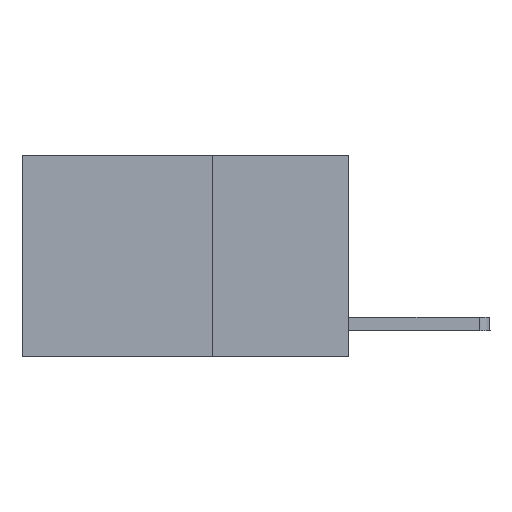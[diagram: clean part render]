
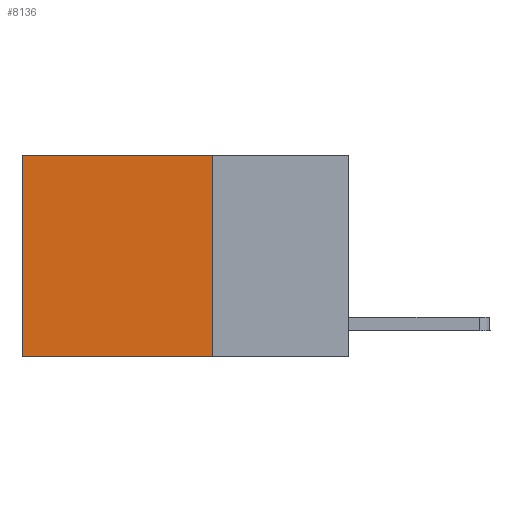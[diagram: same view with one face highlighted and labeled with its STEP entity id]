
A CAD part, left-side view. The second image highlights one B-rep face of the part: STEP entity #8136.
In plain terms, the highlighted planar face has unit normal (-1, 0, 0).
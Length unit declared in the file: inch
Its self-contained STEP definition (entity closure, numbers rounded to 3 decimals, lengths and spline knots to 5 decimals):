
#453 = ORIENTED_EDGE ( 'NONE', *, *, #1893, .F. ) ;
#514 = EDGE_CURVE ( 'NONE', #7480, #708, #1747, .T. ) ;
#708 = VERTEX_POINT ( 'NONE', #3586 ) ;
#758 = DIRECTION ( 'NONE',  ( 0., 1., 0. ) ) ;
#952 = CARTESIAN_POINT ( 'NONE',  ( 0.2625, 0.6, 0. ) ) ;
#1165 = VERTEX_POINT ( 'NONE', #2526 ) ;
#1647 = VERTEX_POINT ( 'NONE', #8555 ) ;
#1747 = LINE ( 'NONE', #3831, #3969 ) ;
#1850 = VECTOR ( 'NONE', #7423, 39.37008 ) ;
#1893 = EDGE_CURVE ( 'NONE', #1647, #1165, #5089, .T. ) ;
#1914 = CARTESIAN_POINT ( 'NONE',  ( 0.2625, 0.25, 0. ) ) ;
#2224 = LINE ( 'NONE', #7095, #2429 ) ;
#2429 = VECTOR ( 'NONE', #758, 39.37008 ) ;
#2526 = CARTESIAN_POINT ( 'NONE',  ( 0.2625, 0.25, -0.37 ) ) ;
#2721 = ORIENTED_EDGE ( 'NONE', *, *, #7191, .T. ) ;
#2847 = DIRECTION ( 'NONE',  ( 0., 0., -1. ) ) ;
#3586 = CARTESIAN_POINT ( 'NONE',  ( 0.2625, 0.6, -0.37 ) ) ;
#3684 = AXIS2_PLACEMENT_3D ( 'NONE', #4658, #7425, #4567 ) ;
#3831 = CARTESIAN_POINT ( 'NONE',  ( 0.2625, 0.6, 0. ) ) ;
#3880 = DIRECTION ( 'NONE',  ( 0., 0., -1. ) ) ;
#3969 = VECTOR ( 'NONE', #3880, 39.37008 ) ;
#4227 = ORIENTED_EDGE ( 'NONE', *, *, #8881, .F. ) ;
#4567 = DIRECTION ( 'NONE',  ( 0., 0., -1. ) ) ;
#4658 = CARTESIAN_POINT ( 'NONE',  ( 0.2625, 0.25, 0. ) ) ;
#5089 = LINE ( 'NONE', #5870, #6672 ) ;
#5213 = LINE ( 'NONE', #1914, #1850 ) ;
#5215 = FACE_OUTER_BOUND ( 'NONE', #6217, .T. ) ;
#5870 = CARTESIAN_POINT ( 'NONE',  ( 0.2625, 0.25, 0. ) ) ;
#6074 = ORIENTED_EDGE ( 'NONE', *, *, #514, .T. ) ;
#6217 = EDGE_LOOP ( 'NONE', ( #6074, #4227, #453, #2721 ) ) ;
#6672 = VECTOR ( 'NONE', #2847, 39.37008 ) ;
#7095 = CARTESIAN_POINT ( 'NONE',  ( 0.2625, 0.25, -0.37 ) ) ;
#7191 = EDGE_CURVE ( 'NONE', #1647, #7480, #5213, .T. ) ;
#7388 = PLANE ( 'NONE',  #3684 ) ;
#7423 = DIRECTION ( 'NONE',  ( 0., 1., 0. ) ) ;
#7425 = DIRECTION ( 'NONE',  ( 1., 0., 0. ) ) ;
#7480 = VERTEX_POINT ( 'NONE', #952 ) ;
#8136 = ADVANCED_FACE ( 'NONE', ( #5215 ), #7388, .F. ) ;
#8555 = CARTESIAN_POINT ( 'NONE',  ( 0.2625, 0.25, 0. ) ) ;
#8881 = EDGE_CURVE ( 'NONE', #1165, #708, #2224, .T. ) ;
